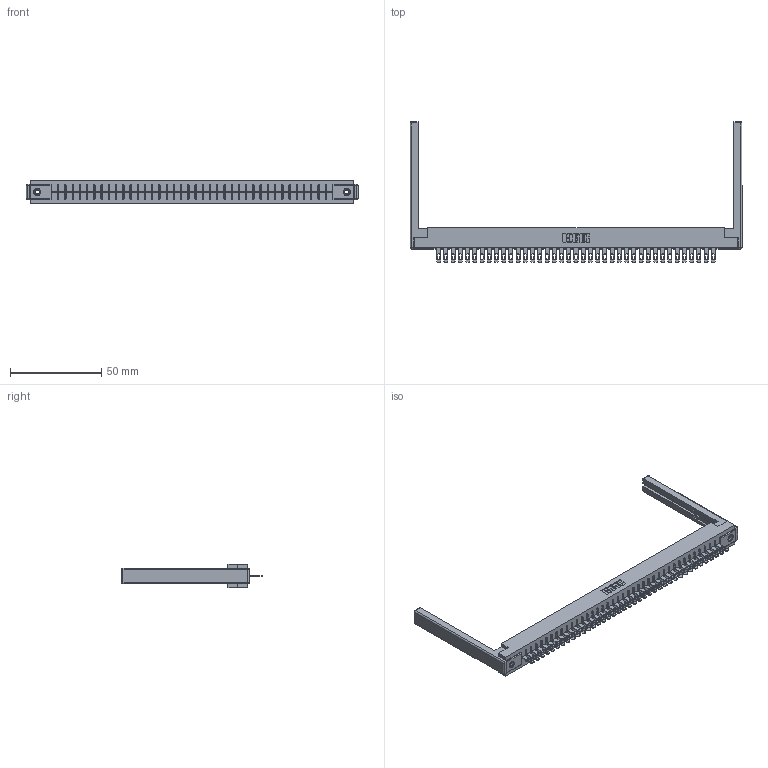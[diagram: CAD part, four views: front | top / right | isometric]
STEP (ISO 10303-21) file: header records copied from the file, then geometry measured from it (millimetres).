
FILE_DESCRIPTION (( 'STEP AP203' ), '1' );
FILE_NAME ('306-039-500-168.STEP', '2019-09-12T00:07:42', ( '' ), ( '' ), 'SwSTEP 2.0', 'SolidWorks 2016', '' );
FILE_SCHEMA (( 'CONFIG_CONTROL_DESIGN' ));
Length unit declared in the file: inch
Products named in the file (5): 306-290-001_100; 345-250-001_345-250-001-102; 306-039-500-168; 307-220-068; 306 Part_.156 Dia
Assembly tree (44 placements, depth 2):
  306-039-500-168
    306 Part_.156 Dia
    306-290-001_100  x39
    345-250-001_345-250-001-102  x2
    307-220-068  x2
Bounding box: 181.97 x 77.17 x 12.7 mm (x, y, z)
Volume: 24582.7 mm3; surface area: 25471.5 mm2
Topology: 44 solids, 44 shells, 3234 faces, 9091 edges, 5830 vertices
Faces by surface type: plane 2106, cylinder 948, sphere 164, cone 12, torus 4
Entity records: 39681 total; most frequent: CARTESIAN_POINT 6629, ORIENTED_EDGE 6564, DIRECTION 6550, EDGE_CURVE 3282, VECTOR 2560, LINE 2560, VERTEX_POINT 2074, AXIS2_PLACEMENT_3D 1995
